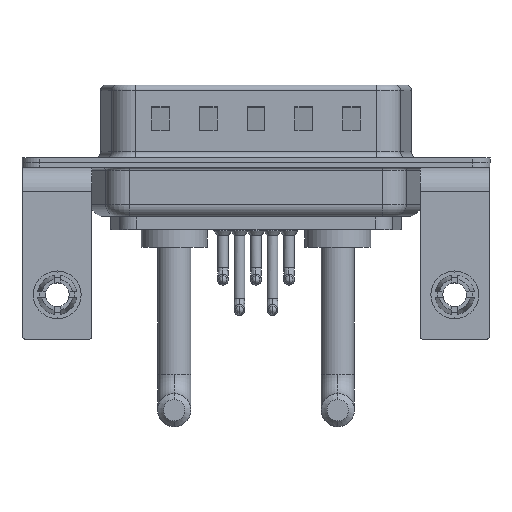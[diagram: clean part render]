
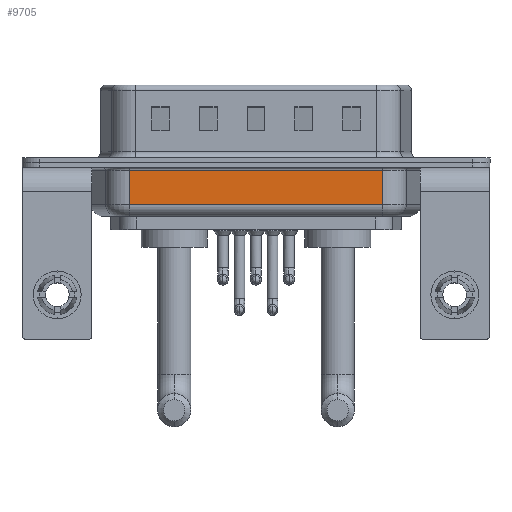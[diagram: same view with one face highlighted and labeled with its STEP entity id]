
A CAD part, front view. The second image highlights one B-rep face of the part: STEP entity #9705.
In plain terms, the highlighted planar face has unit normal (0, -1, 0).
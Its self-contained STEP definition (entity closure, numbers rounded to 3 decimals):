
#899 = DIRECTION ( 'NONE',  ( 0., 1., 0. ) ) ;
#1433 = CARTESIAN_POINT ( 'NONE',  ( 27.269, -5.35, -3.5 ) ) ;
#1881 = VERTEX_POINT ( 'NONE', #19067 ) ;
#2707 = LINE ( 'NONE', #11610, #18748 ) ;
#2967 = ORIENTED_EDGE ( 'NONE', *, *, #13623, .T. ) ;
#3832 = EDGE_CURVE ( 'NONE', #19443, #19801, #16152, .T. ) ;
#3873 = VERTEX_POINT ( 'NONE', #12610 ) ;
#5394 = DIRECTION ( 'NONE',  ( 0., 0., 1. ) ) ;
#6353 = LINE ( 'NONE', #13360, #22383 ) ;
#6368 = PLANE ( 'NONE',  #22329 ) ;
#6817 = CARTESIAN_POINT ( 'NONE',  ( 27.269, -5.35, -4.5 ) ) ;
#8586 = LINE ( 'NONE', #6817, #12217 ) ;
#9705 = ADVANCED_FACE ( 'NONE', ( #19183 ), #6368, .F. ) ;
#11375 = CARTESIAN_POINT ( 'NONE',  ( 6.031, -5.35, -3.5 ) ) ;
#11610 = CARTESIAN_POINT ( 'NONE',  ( 6.031, -5.35, -0.65 ) ) ;
#11727 = DIRECTION ( 'NONE',  ( -1., 0., 0. ) ) ;
#12217 = VECTOR ( 'NONE', #5394, 1000. ) ;
#12423 = ORIENTED_EDGE ( 'NONE', *, *, #17721, .T. ) ;
#12610 = CARTESIAN_POINT ( 'NONE',  ( 6.031, -5.35, -0.65 ) ) ;
#13360 = CARTESIAN_POINT ( 'NONE',  ( 6.031, -5.35, -4.5 ) ) ;
#13623 = EDGE_CURVE ( 'NONE', #19801, #1881, #8586, .T. ) ;
#13855 = CARTESIAN_POINT ( 'NONE',  ( 6.031, -5.35, -4.5 ) ) ;
#14738 = DIRECTION ( 'NONE',  ( 1., 0., 0. ) ) ;
#15393 = EDGE_LOOP ( 'NONE', ( #15635, #17734, #2967, #12423 ) ) ;
#15635 = ORIENTED_EDGE ( 'NONE', *, *, #21254, .F. ) ;
#16152 = LINE ( 'NONE', #20222, #18018 ) ;
#17376 = DIRECTION ( 'NONE',  ( 0., 0., 1. ) ) ;
#17635 = DIRECTION ( 'NONE',  ( 0., 0., 1. ) ) ;
#17721 = EDGE_CURVE ( 'NONE', #1881, #3873, #2707, .T. ) ;
#17734 = ORIENTED_EDGE ( 'NONE', *, *, #3832, .T. ) ;
#18018 = VECTOR ( 'NONE', #14738, 1000. ) ;
#18748 = VECTOR ( 'NONE', #11727, 1000. ) ;
#19067 = CARTESIAN_POINT ( 'NONE',  ( 27.269, -5.35, -0.65 ) ) ;
#19183 = FACE_OUTER_BOUND ( 'NONE', #15393, .T. ) ;
#19443 = VERTEX_POINT ( 'NONE', #11375 ) ;
#19801 = VERTEX_POINT ( 'NONE', #1433 ) ;
#20222 = CARTESIAN_POINT ( 'NONE',  ( 6.031, -5.35, -3.5 ) ) ;
#21254 = EDGE_CURVE ( 'NONE', #19443, #3873, #6353, .T. ) ;
#22329 = AXIS2_PLACEMENT_3D ( 'NONE', #13855, #899, #17635 ) ;
#22383 = VECTOR ( 'NONE', #17376, 1000. ) ;
